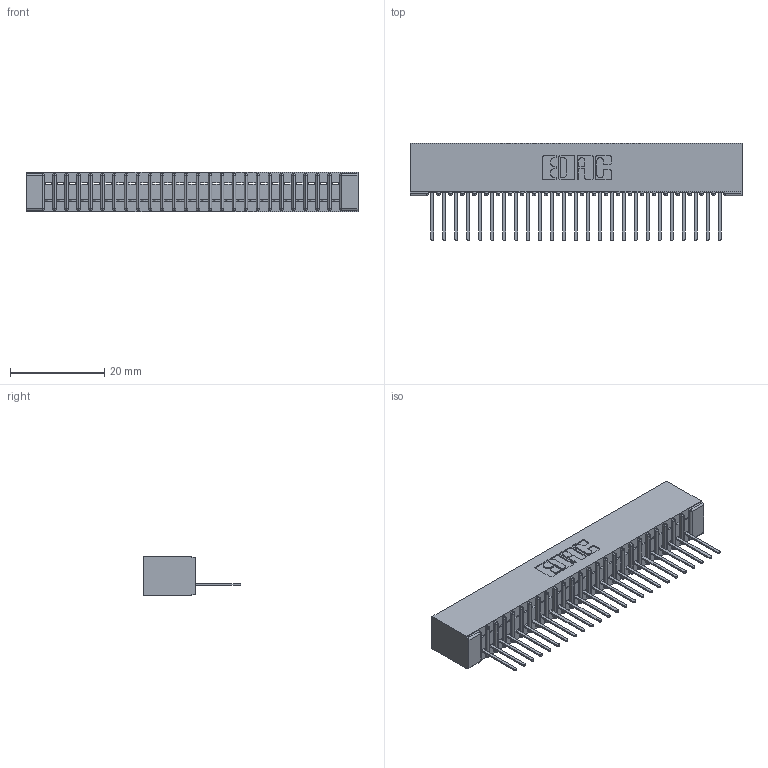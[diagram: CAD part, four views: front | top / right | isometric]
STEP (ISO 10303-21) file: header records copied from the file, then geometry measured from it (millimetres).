
FILE_DESCRIPTION (( 'STEP AP203' ), '1' );
FILE_NAME ('391-025-522-101.STEP', '2018-08-08T20:07:22', ( '' ), ( '' ), 'SwSTEP 2.0', 'SolidWorks 2016', '' );
FILE_SCHEMA (( 'CONFIG_CONTROL_DESIGN' ));
Length unit declared in the file: inch
Products named in the file (3): 341 Part_No Mounting Lugs; 341-292-001_341-292-122; 391-025-522-101
Assembly tree (26 placements, depth 2):
  391-025-522-101
    341 Part_No Mounting Lugs
    341-292-001_341-292-122  x25
Bounding box: 70.48 x 20.62 x 8.38 mm (x, y, z)
Volume: 3988.8 mm3; surface area: 8192 mm2
Topology: 26 solids, 26 shells, 2158 faces, 6217 edges, 3990 vertices
Faces by surface type: plane 1339, cylinder 719, sphere 52, torus 48
Entity records: 31442 total; most frequent: CARTESIAN_POINT 5334, ORIENTED_EDGE 5322, DIRECTION 5161, EDGE_CURVE 2661, VECTOR 2135, LINE 2135, VERTEX_POINT 1686, AXIS2_PLACEMENT_3D 1513
